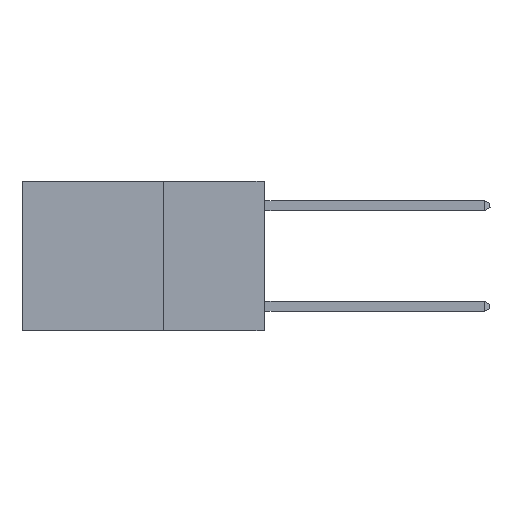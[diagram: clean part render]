
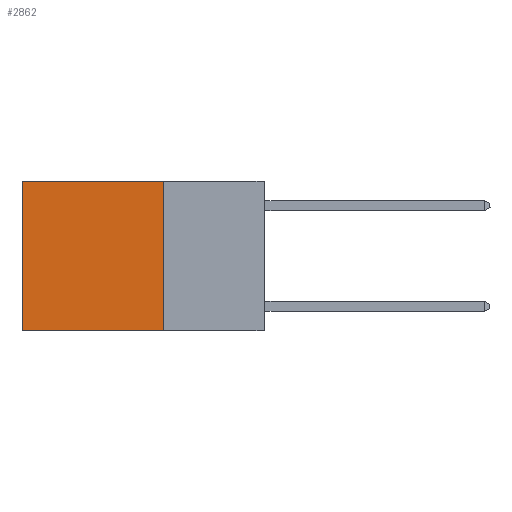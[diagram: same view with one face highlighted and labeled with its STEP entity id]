
A CAD part, left-side view. The second image highlights one B-rep face of the part: STEP entity #2862.
In plain terms, the highlighted planar face has unit normal (-1, 0, 0).
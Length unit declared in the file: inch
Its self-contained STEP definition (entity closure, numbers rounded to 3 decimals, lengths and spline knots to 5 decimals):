
#417 = EDGE_CURVE ( 'NONE', #12860, #20311, #17579, .T. ) ;
#1409 = VECTOR ( 'NONE', #3919, 39.37008 ) ;
#2862 = ADVANCED_FACE ( 'NONE', ( #7328 ), #20426, .F. ) ;
#3919 = DIRECTION ( 'NONE',  ( 0., 0., -1. ) ) ;
#4442 = AXIS2_PLACEMENT_3D ( 'NONE', #7381, #9173, #7452 ) ;
#4587 = EDGE_CURVE ( 'NONE', #11514, #8793, #8063, .T. ) ;
#5305 = DIRECTION ( 'NONE',  ( 0., 1., 0. ) ) ;
#6153 = DIRECTION ( 'NONE',  ( 0., 0., -1. ) ) ;
#7250 = ORIENTED_EDGE ( 'NONE', *, *, #4587, .T. ) ;
#7328 = FACE_OUTER_BOUND ( 'NONE', #17548, .T. ) ;
#7347 = LINE ( 'NONE', #8517, #21218 ) ;
#7381 = CARTESIAN_POINT ( 'NONE',  ( 0.2625, 0.25, 0. ) ) ;
#7452 = DIRECTION ( 'NONE',  ( 0., 0., -1. ) ) ;
#7538 = VECTOR ( 'NONE', #6153, 39.37008 ) ;
#8063 = LINE ( 'NONE', #9328, #7538 ) ;
#8443 = DIRECTION ( 'NONE',  ( 0., 1., 0. ) ) ;
#8517 = CARTESIAN_POINT ( 'NONE',  ( 0.2625, 0.25, 0. ) ) ;
#8765 = ORIENTED_EDGE ( 'NONE', *, *, #19415, .T. ) ;
#8793 = VERTEX_POINT ( 'NONE', #17276 ) ;
#8865 = LINE ( 'NONE', #13239, #16333 ) ;
#9173 = DIRECTION ( 'NONE',  ( 1., 0., 0. ) ) ;
#9328 = CARTESIAN_POINT ( 'NONE',  ( 0.2625, 0.6, 0. ) ) ;
#10492 = CARTESIAN_POINT ( 'NONE',  ( 0.2625, 0.25, -0.37 ) ) ;
#10508 = CARTESIAN_POINT ( 'NONE',  ( 0.2625, 0.25, 0. ) ) ;
#10797 = EDGE_CURVE ( 'NONE', #20311, #8793, #8865, .T. ) ;
#11514 = VERTEX_POINT ( 'NONE', #20067 ) ;
#12860 = VERTEX_POINT ( 'NONE', #20988 ) ;
#13239 = CARTESIAN_POINT ( 'NONE',  ( 0.2625, 0.25, -0.37 ) ) ;
#16333 = VECTOR ( 'NONE', #5305, 39.37008 ) ;
#17276 = CARTESIAN_POINT ( 'NONE',  ( 0.2625, 0.6, -0.37 ) ) ;
#17510 = ORIENTED_EDGE ( 'NONE', *, *, #417, .F. ) ;
#17548 = EDGE_LOOP ( 'NONE', ( #7250, #18934, #17510, #8765 ) ) ;
#17579 = LINE ( 'NONE', #10508, #1409 ) ;
#18934 = ORIENTED_EDGE ( 'NONE', *, *, #10797, .F. ) ;
#19415 = EDGE_CURVE ( 'NONE', #12860, #11514, #7347, .T. ) ;
#20067 = CARTESIAN_POINT ( 'NONE',  ( 0.2625, 0.6, 0. ) ) ;
#20311 = VERTEX_POINT ( 'NONE', #10492 ) ;
#20426 = PLANE ( 'NONE',  #4442 ) ;
#20988 = CARTESIAN_POINT ( 'NONE',  ( 0.2625, 0.25, 0. ) ) ;
#21218 = VECTOR ( 'NONE', #8443, 39.37008 ) ;
